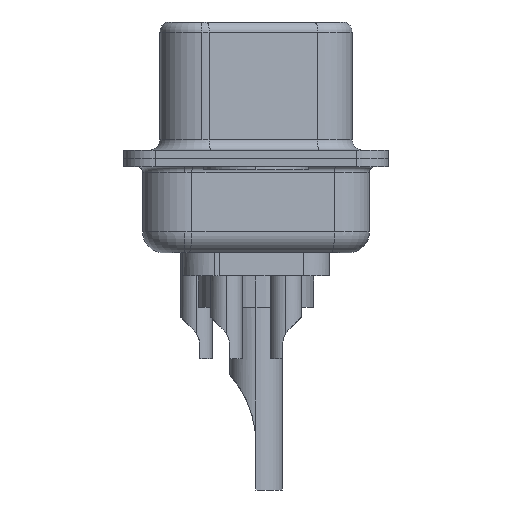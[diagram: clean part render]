
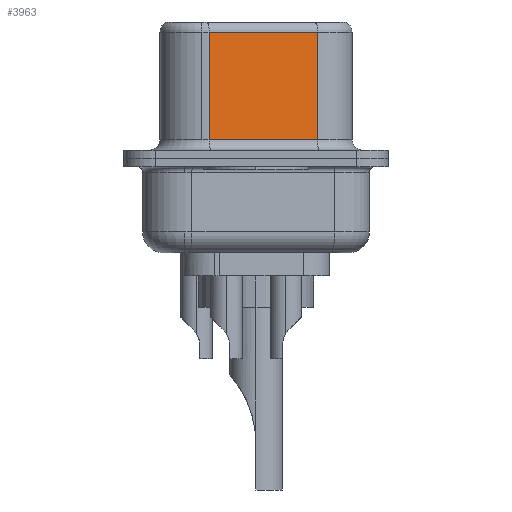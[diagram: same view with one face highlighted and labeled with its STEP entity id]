
A CAD part, left-side view. The second image highlights one B-rep face of the part: STEP entity #3963.
In plain terms, the highlighted planar face has unit normal (-0.985, -0.174, 0).
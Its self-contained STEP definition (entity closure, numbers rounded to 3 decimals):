
#136 = CARTESIAN_POINT ( 'NONE',  ( 4.585, -2.927, 6.02 ) ) ;
#1756 = DIRECTION ( 'NONE',  ( -0.174, 0.985, 0. ) ) ;
#2136 = CARTESIAN_POINT ( 'NONE',  ( 3.675, 2.233, 0.9 ) ) ;
#2467 = DIRECTION ( 'NONE',  ( 0.174, -0.985, 0. ) ) ;
#2752 = VERTEX_POINT ( 'NONE', #5767 ) ;
#2955 = ORIENTED_EDGE ( 'NONE', *, *, #12959, .T. ) ;
#3902 = VERTEX_POINT ( 'NONE', #14321 ) ;
#3963 = ADVANCED_FACE ( 'NONE', ( #18731 ), #13513, .F. ) ;
#4365 = VERTEX_POINT ( 'NONE', #2136 ) ;
#5026 = EDGE_CURVE ( 'NONE', #16287, #3902, #12489, .T. ) ;
#5074 = AXIS2_PLACEMENT_3D ( 'NONE', #9228, #16322, #17790 ) ;
#5383 = CARTESIAN_POINT ( 'NONE',  ( 4.585, -2.927, 0.9 ) ) ;
#5585 = CARTESIAN_POINT ( 'NONE',  ( 4.585, -2.927, 6.52 ) ) ;
#5767 = CARTESIAN_POINT ( 'NONE',  ( 3.675, 2.233, 6.02 ) ) ;
#5880 = DIRECTION ( 'NONE',  ( 0., 0., -1. ) ) ;
#8283 = VECTOR ( 'NONE', #9947, 1000. ) ;
#8638 = ORIENTED_EDGE ( 'NONE', *, *, #10701, .T. ) ;
#8963 = CARTESIAN_POINT ( 'NONE',  ( 4.585, -2.927, 6.02 ) ) ;
#9228 = CARTESIAN_POINT ( 'NONE',  ( 4.585, -2.927, 6.52 ) ) ;
#9525 = EDGE_CURVE ( 'NONE', #16287, #2752, #17597, .T. ) ;
#9947 = DIRECTION ( 'NONE',  ( 0., 0., -1. ) ) ;
#10701 = EDGE_CURVE ( 'NONE', #4365, #3902, #18056, .T. ) ;
#12174 = CARTESIAN_POINT ( 'NONE',  ( 3.675, 2.233, 6.52 ) ) ;
#12489 = LINE ( 'NONE', #5585, #8283 ) ;
#12959 = EDGE_CURVE ( 'NONE', #2752, #4365, #17974, .T. ) ;
#13015 = VECTOR ( 'NONE', #1756, 1000. ) ;
#13349 = ORIENTED_EDGE ( 'NONE', *, *, #9525, .T. ) ;
#13513 = PLANE ( 'NONE',  #5074 ) ;
#14321 = CARTESIAN_POINT ( 'NONE',  ( 4.585, -2.927, 0.9 ) ) ;
#15046 = ORIENTED_EDGE ( 'NONE', *, *, #5026, .F. ) ;
#16088 = EDGE_LOOP ( 'NONE', ( #15046, #13349, #2955, #8638 ) ) ;
#16287 = VERTEX_POINT ( 'NONE', #8963 ) ;
#16322 = DIRECTION ( 'NONE',  ( 0.985, 0.174, 0. ) ) ;
#17098 = VECTOR ( 'NONE', #2467, 1000. ) ;
#17498 = VECTOR ( 'NONE', #5880, 1000. ) ;
#17597 = LINE ( 'NONE', #136, #13015 ) ;
#17790 = DIRECTION ( 'NONE',  ( -0.174, 0.985, 0. ) ) ;
#17974 = LINE ( 'NONE', #12174, #17498 ) ;
#18056 = LINE ( 'NONE', #5383, #17098 ) ;
#18731 = FACE_OUTER_BOUND ( 'NONE', #16088, .T. ) ;
